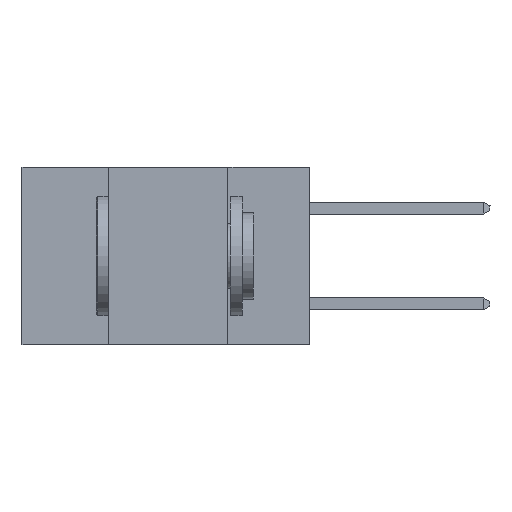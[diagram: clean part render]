
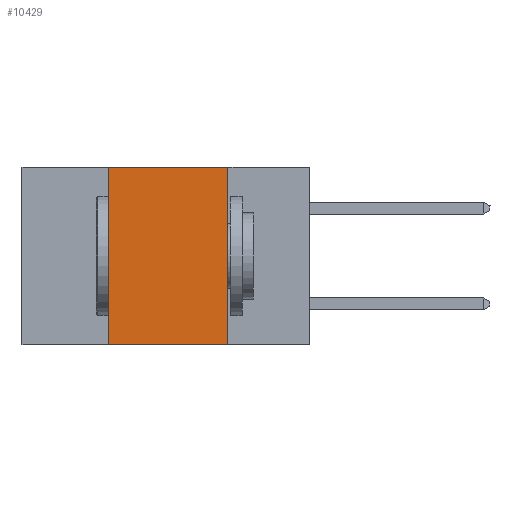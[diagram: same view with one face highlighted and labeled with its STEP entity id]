
A CAD part, left-side view. The second image highlights one B-rep face of the part: STEP entity #10429.
In plain terms, the highlighted planar face has unit normal (-1, 0, 0).
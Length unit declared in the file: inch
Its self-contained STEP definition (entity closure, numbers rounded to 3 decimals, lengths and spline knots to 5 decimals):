
#1067 = CARTESIAN_POINT ( 'NONE',  ( 0., 0.42, 0. ) ) ;
#1079 = EDGE_CURVE ( 'NONE', #7227, #2991, #13293, .T. ) ;
#2182 = CARTESIAN_POINT ( 'NONE',  ( 0., 0.6, 0. ) ) ;
#2991 = VERTEX_POINT ( 'NONE', #16152 ) ;
#3790 = DIRECTION ( 'NONE',  ( 1., 0., 0. ) ) ;
#4254 = DIRECTION ( 'NONE',  ( 0., -1., 0. ) ) ;
#4269 = DIRECTION ( 'NONE',  ( 0., 0., 1. ) ) ;
#4779 = ORIENTED_EDGE ( 'NONE', *, *, #1079, .F. ) ;
#5113 = VECTOR ( 'NONE', #4254, 39.37008 ) ;
#5219 = CARTESIAN_POINT ( 'NONE',  ( 0., 0.6, -0.37 ) ) ;
#6141 = LINE ( 'NONE', #5219, #10254 ) ;
#6369 = EDGE_CURVE ( 'NONE', #15523, #7227, #12710, .T. ) ;
#7012 = VERTEX_POINT ( 'NONE', #11881 ) ;
#7130 = CARTESIAN_POINT ( 'NONE',  ( 0., 0.6, 0. ) ) ;
#7145 = CARTESIAN_POINT ( 'NONE',  ( 0., 0.17, 0. ) ) ;
#7227 = VERTEX_POINT ( 'NONE', #7787 ) ;
#7498 = EDGE_LOOP ( 'NONE', ( #16516, #4779, #15372, #15458 ) ) ;
#7541 = VECTOR ( 'NONE', #10245, 39.37008 ) ;
#7787 = CARTESIAN_POINT ( 'NONE',  ( 0., 0.42, 0. ) ) ;
#8174 = VECTOR ( 'NONE', #4269, 39.37008 ) ;
#8440 = CARTESIAN_POINT ( 'NONE',  ( 0., 0.42, -0.37 ) ) ;
#9907 = DIRECTION ( 'NONE',  ( 0., -1., 0. ) ) ;
#10245 = DIRECTION ( 'NONE',  ( 0., 0., -1. ) ) ;
#10254 = VECTOR ( 'NONE', #9907, 39.37008 ) ;
#10429 = ADVANCED_FACE ( 'NONE', ( #18113 ), #11519, .F. ) ;
#10529 = EDGE_CURVE ( 'NONE', #2991, #7012, #16182, .T. ) ;
#11519 = PLANE ( 'NONE',  #18990 ) ;
#11881 = CARTESIAN_POINT ( 'NONE',  ( 0., 0.17, -0.37 ) ) ;
#12710 = LINE ( 'NONE', #1067, #8174 ) ;
#13293 = LINE ( 'NONE', #7130, #5113 ) ;
#13937 = EDGE_CURVE ( 'NONE', #15523, #7012, #6141, .T. ) ;
#14557 = DIRECTION ( 'NONE',  ( 0., 0., -1. ) ) ;
#15372 = ORIENTED_EDGE ( 'NONE', *, *, #6369, .F. ) ;
#15458 = ORIENTED_EDGE ( 'NONE', *, *, #13937, .T. ) ;
#15523 = VERTEX_POINT ( 'NONE', #8440 ) ;
#16152 = CARTESIAN_POINT ( 'NONE',  ( 0., 0.17, 0. ) ) ;
#16182 = LINE ( 'NONE', #7145, #7541 ) ;
#16516 = ORIENTED_EDGE ( 'NONE', *, *, #10529, .F. ) ;
#18113 = FACE_OUTER_BOUND ( 'NONE', #7498, .T. ) ;
#18990 = AXIS2_PLACEMENT_3D ( 'NONE', #2182, #3790, #14557 ) ;
